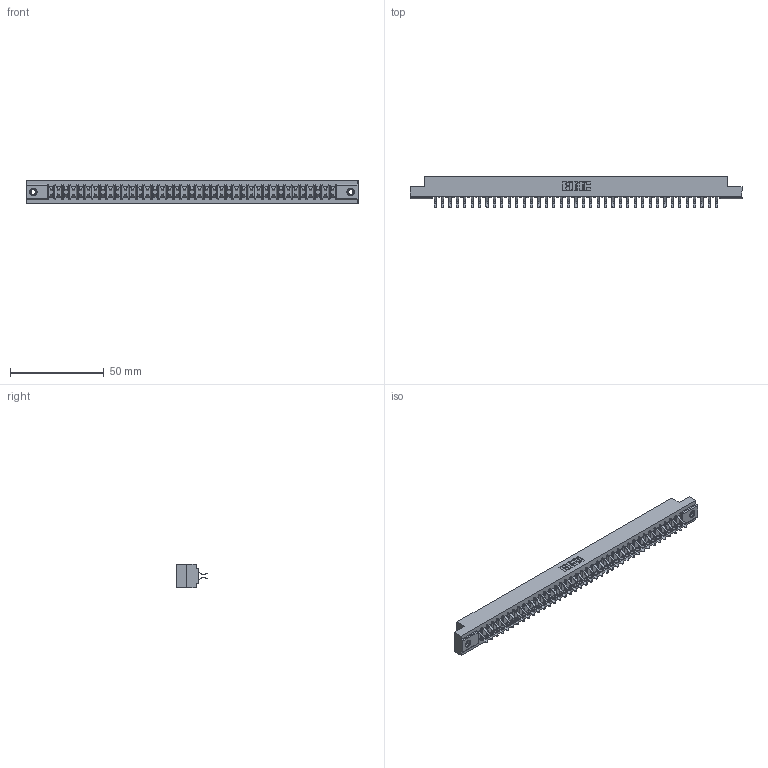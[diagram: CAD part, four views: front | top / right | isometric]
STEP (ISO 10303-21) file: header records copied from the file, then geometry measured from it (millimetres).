
FILE_DESCRIPTION (( 'STEP AP203' ), '1' );
FILE_NAME ('357-078-556-207.STEP', '2018-08-12T22:42:03', ( '' ), ( '' ), 'SwSTEP 2.0', 'SolidWorks 2016', '' );
FILE_SCHEMA (( 'CONFIG_CONTROL_DESIGN' ));
Length unit declared in the file: inch
Products named in the file (4): 307 Part_.156 Dia Mounting Holes; 307-290-001_556; 345-250-001_345-250-005-103; 357-078-556-207
Assembly tree (81 placements, depth 2):
  357-078-556-207
    307 Part_.156 Dia Mounting Holes
    307-290-001_556  x78
    345-250-001_345-250-005-103  x2
Bounding box: 177.55 x 16.97 x 12.7 mm (x, y, z)
Volume: 18831 mm3; surface area: 22808.1 mm2
Topology: 81 solids, 81 shells, 4118 faces, 11535 edges, 7470 vertices
Faces by surface type: plane 2676, cylinder 1346, sphere 80, cone 12, torus 4
Entity records: 36341 total; most frequent: CARTESIAN_POINT 5930, ORIENTED_EDGE 5870, DIRECTION 5819, EDGE_CURVE 2935, LINE 2249, VECTOR 2249, VERTEX_POINT 1896, AXIS2_PLACEMENT_3D 1785
